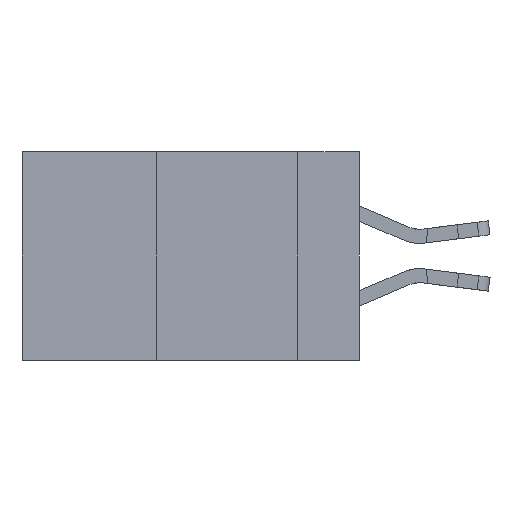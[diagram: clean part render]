
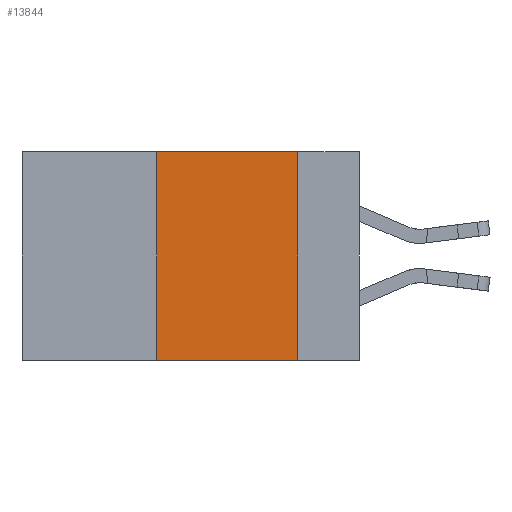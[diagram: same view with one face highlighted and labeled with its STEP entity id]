
A CAD part, left-side view. The second image highlights one B-rep face of the part: STEP entity #13844.
In plain terms, the highlighted planar face has unit normal (-1, 0, 0).
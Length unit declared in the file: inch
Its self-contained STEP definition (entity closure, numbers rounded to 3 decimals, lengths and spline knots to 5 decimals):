
#520 = VECTOR ( 'NONE', #2339, 39.37008 ) ;
#1088 = VERTEX_POINT ( 'NONE', #5986 ) ;
#1668 = VECTOR ( 'NONE', #15338, 39.37008 ) ;
#2029 = LINE ( 'NONE', #10900, #15285 ) ;
#2339 = DIRECTION ( 'NONE',  ( 0., -1., 0. ) ) ;
#3308 = FACE_OUTER_BOUND ( 'NONE', #5230, .T. ) ;
#3639 = EDGE_CURVE ( 'NONE', #1088, #11683, #6499, .T. ) ;
#5230 = EDGE_LOOP ( 'NONE', ( #21840, #9627, #6179, #11165 ) ) ;
#5263 = DIRECTION ( 'NONE',  ( 1., 0., 0. ) ) ;
#5986 = CARTESIAN_POINT ( 'NONE',  ( 0., 0.36, 0. ) ) ;
#6116 = EDGE_CURVE ( 'NONE', #11683, #6134, #2029, .T. ) ;
#6122 = EDGE_CURVE ( 'NONE', #17473, #1088, #10612, .T. ) ;
#6134 = VERTEX_POINT ( 'NONE', #9104 ) ;
#6179 = ORIENTED_EDGE ( 'NONE', *, *, #6122, .F. ) ;
#6329 = EDGE_CURVE ( 'NONE', #17473, #6134, #14997, .T. ) ;
#6499 = LINE ( 'NONE', #8386, #1668 ) ;
#8386 = CARTESIAN_POINT ( 'NONE',  ( 0., 0.6, 0. ) ) ;
#8910 = CARTESIAN_POINT ( 'NONE',  ( 0., 0.6, 0. ) ) ;
#9020 = DIRECTION ( 'NONE',  ( 0., 0., -1. ) ) ;
#9104 = CARTESIAN_POINT ( 'NONE',  ( 0., 0.11, -0.37 ) ) ;
#9627 = ORIENTED_EDGE ( 'NONE', *, *, #3639, .F. ) ;
#10612 = LINE ( 'NONE', #17912, #19289 ) ;
#10707 = PLANE ( 'NONE',  #17106 ) ;
#10900 = CARTESIAN_POINT ( 'NONE',  ( 0., 0.11, 0. ) ) ;
#11165 = ORIENTED_EDGE ( 'NONE', *, *, #6329, .T. ) ;
#11683 = VERTEX_POINT ( 'NONE', #16515 ) ;
#13844 = ADVANCED_FACE ( 'NONE', ( #3308 ), #10707, .F. ) ;
#14997 = LINE ( 'NONE', #21657, #520 ) ;
#15285 = VECTOR ( 'NONE', #9020, 39.37008 ) ;
#15338 = DIRECTION ( 'NONE',  ( 0., -1., 0. ) ) ;
#16515 = CARTESIAN_POINT ( 'NONE',  ( 0., 0.11, 0. ) ) ;
#17106 = AXIS2_PLACEMENT_3D ( 'NONE', #8910, #5263, #17735 ) ;
#17473 = VERTEX_POINT ( 'NONE', #21150 ) ;
#17735 = DIRECTION ( 'NONE',  ( 0., 0., -1. ) ) ;
#17912 = CARTESIAN_POINT ( 'NONE',  ( 0., 0.36, 0. ) ) ;
#19289 = VECTOR ( 'NONE', #19556, 39.37008 ) ;
#19556 = DIRECTION ( 'NONE',  ( 0., 0., 1. ) ) ;
#21150 = CARTESIAN_POINT ( 'NONE',  ( 0., 0.36, -0.37 ) ) ;
#21657 = CARTESIAN_POINT ( 'NONE',  ( 0., 0.6, -0.37 ) ) ;
#21840 = ORIENTED_EDGE ( 'NONE', *, *, #6116, .F. ) ;
